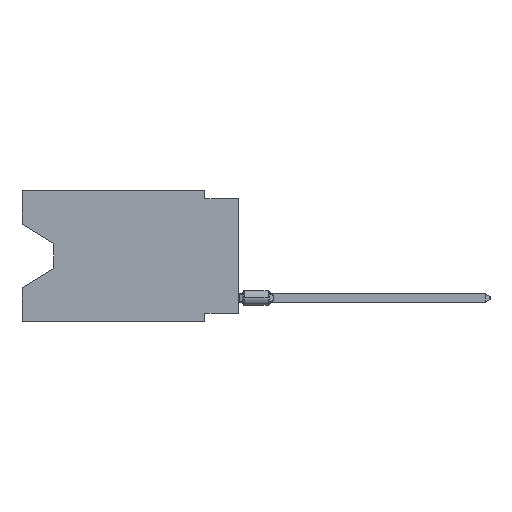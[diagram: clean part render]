
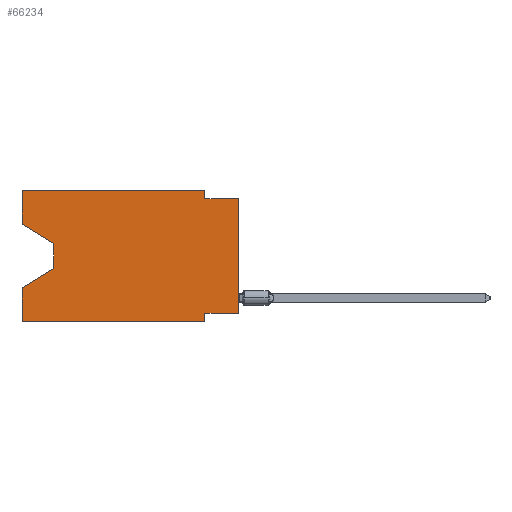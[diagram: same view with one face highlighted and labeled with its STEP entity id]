
A CAD part, left-side view. The second image highlights one B-rep face of the part: STEP entity #66234.
In plain terms, the highlighted planar face has unit normal (-1, 0, 0).
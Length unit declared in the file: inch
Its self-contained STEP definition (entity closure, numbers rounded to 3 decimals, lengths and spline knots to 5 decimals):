
#13 = DIRECTION ( 'NONE',  ( 0., -0.855, -0.519 ) ) ;
#1973 = DIRECTION ( 'NONE',  ( 0., -1., 0. ) ) ;
#2079 = EDGE_CURVE ( 'NONE', #6070, #27769, #16636, .T. ) ;
#2170 = EDGE_CURVE ( 'NONE', #6070, #48036, #61085, .T. ) ;
#4912 = DIRECTION ( 'NONE',  ( 0., 0., 1. ) ) ;
#6001 = CARTESIAN_POINT ( 'NONE',  ( 0., 0., 0. ) ) ;
#6070 = VERTEX_POINT ( 'NONE', #34363 ) ;
#8718 = CARTESIAN_POINT ( 'NONE',  ( 0., 0.645, 0. ) ) ;
#9773 = DIRECTION ( 'NONE',  ( 0., -1., 0. ) ) ;
#10427 = VECTOR ( 'NONE', #58293, 39.37008 ) ;
#11369 = CARTESIAN_POINT ( 'NONE',  ( 0., 0.645, -0.10025 ) ) ;
#11467 = DIRECTION ( 'NONE',  ( 0., 1., 0. ) ) ;
#11790 = VERTEX_POINT ( 'NONE', #64681 ) ;
#13899 = CARTESIAN_POINT ( 'NONE',  ( 0., 0., -0.025 ) ) ;
#14241 = LINE ( 'NONE', #26767, #72874 ) ;
#14348 = VERTEX_POINT ( 'NONE', #54433 ) ;
#14787 = VERTEX_POINT ( 'NONE', #48953 ) ;
#14793 = FACE_OUTER_BOUND ( 'NONE', #17022, .T. ) ;
#14929 = DIRECTION ( 'NONE',  ( 0., 0., -1. ) ) ;
#15572 = DIRECTION ( 'NONE',  ( 0., 0., -1. ) ) ;
#16636 = LINE ( 'NONE', #78474, #10427 ) ;
#16924 = DIRECTION ( 'NONE',  ( 0., 0., 1. ) ) ;
#17022 = EDGE_LOOP ( 'NONE', ( #77737, #52090, #46063, #29889, #41522, #38681, #74377, #63121, #40506, #45290, #59049, #35788 ) ) ;
#21013 = DIRECTION ( 'NONE',  ( 0., 0., -1. ) ) ;
#21389 = EDGE_CURVE ( 'NONE', #25518, #65332, #34711, .T. ) ;
#23384 = VECTOR ( 'NONE', #11467, 39.37008 ) ;
#24010 = CARTESIAN_POINT ( 'NONE',  ( 0., 0., -0.365 ) ) ;
#24041 = CARTESIAN_POINT ( 'NONE',  ( 0., 0., -0.365 ) ) ;
#25518 = VERTEX_POINT ( 'NONE', #32060 ) ;
#26013 = DIRECTION ( 'NONE',  ( 0., -1., 0. ) ) ;
#26548 = VERTEX_POINT ( 'NONE', #24041 ) ;
#26767 = CARTESIAN_POINT ( 'NONE',  ( 0., 0.645, -0.39 ) ) ;
#27011 = LINE ( 'NONE', #32675, #67946 ) ;
#27769 = VERTEX_POINT ( 'NONE', #66499 ) ;
#29889 = ORIENTED_EDGE ( 'NONE', *, *, #64045, .F. ) ;
#32060 = CARTESIAN_POINT ( 'NONE',  ( 0., 0.1, 0. ) ) ;
#32675 = CARTESIAN_POINT ( 'NONE',  ( 0., 0.645, 0. ) ) ;
#33351 = DIRECTION ( 'NONE',  ( 1., 0., 0. ) ) ;
#33460 = EDGE_CURVE ( 'NONE', #77255, #78059, #77399, .T. ) ;
#34363 = CARTESIAN_POINT ( 'NONE',  ( 0., 0.645, -0.10025 ) ) ;
#34711 = LINE ( 'NONE', #76390, #42936 ) ;
#35319 = CARTESIAN_POINT ( 'NONE',  ( 0., 0.645, -0.28975 ) ) ;
#35788 = ORIENTED_EDGE ( 'NONE', *, *, #2079, .F. ) ;
#37312 = CARTESIAN_POINT ( 'NONE',  ( 0., 0.1, -0.025 ) ) ;
#37750 = EDGE_CURVE ( 'NONE', #27769, #25518, #27011, .T. ) ;
#38680 = VECTOR ( 'NONE', #26013, 39.37008 ) ;
#38681 = ORIENTED_EDGE ( 'NONE', *, *, #68670, .F. ) ;
#39824 = VECTOR ( 'NONE', #4912, 39.37008 ) ;
#40506 = ORIENTED_EDGE ( 'NONE', *, *, #54333, .F. ) ;
#41522 = ORIENTED_EDGE ( 'NONE', *, *, #59738, .T. ) ;
#41677 = LINE ( 'NONE', #66348, #39824 ) ;
#42936 = VECTOR ( 'NONE', #21013, 39.37008 ) ;
#43378 = EDGE_CURVE ( 'NONE', #26548, #14348, #66836, .T. ) ;
#45290 = ORIENTED_EDGE ( 'NONE', *, *, #21389, .F. ) ;
#46063 = ORIENTED_EDGE ( 'NONE', *, *, #33460, .T. ) ;
#46192 = LINE ( 'NONE', #13899, #38680 ) ;
#46269 = DIRECTION ( 'NONE',  ( 0., 0., -1. ) ) ;
#47081 = CARTESIAN_POINT ( 'NONE',  ( 0., 0.55, -0.158 ) ) ;
#47676 = VECTOR ( 'NONE', #63695, 39.37008 ) ;
#48036 = VERTEX_POINT ( 'NONE', #68270 ) ;
#48953 = CARTESIAN_POINT ( 'NONE',  ( 0., 0.1, -0.39 ) ) ;
#51961 = CARTESIAN_POINT ( 'NONE',  ( 0., 0.55, -0.232 ) ) ;
#52090 = ORIENTED_EDGE ( 'NONE', *, *, #62322, .T. ) ;
#52495 = LINE ( 'NONE', #64608, #67225 ) ;
#52533 = CARTESIAN_POINT ( 'NONE',  ( 0., 0.645, -0.39 ) ) ;
#54333 = EDGE_CURVE ( 'NONE', #65332, #11790, #46192, .T. ) ;
#54433 = CARTESIAN_POINT ( 'NONE',  ( 0., 0.1, -0.365 ) ) ;
#54611 = CARTESIAN_POINT ( 'NONE',  ( 0., 0.55, -0.232 ) ) ;
#56183 = VECTOR ( 'NONE', #46269, 39.37008 ) ;
#58293 = DIRECTION ( 'NONE',  ( 0., 0., 1. ) ) ;
#59049 = ORIENTED_EDGE ( 'NONE', *, *, #37750, .F. ) ;
#59738 = EDGE_CURVE ( 'NONE', #61241, #14787, #14241, .T. ) ;
#61085 = LINE ( 'NONE', #11369, #76272 ) ;
#61241 = VERTEX_POINT ( 'NONE', #52533 ) ;
#61379 = LINE ( 'NONE', #6001, #64600 ) ;
#62063 = AXIS2_PLACEMENT_3D ( 'NONE', #8718, #33351, #15572 ) ;
#62322 = EDGE_CURVE ( 'NONE', #48036, #77255, #78584, .T. ) ;
#63121 = ORIENTED_EDGE ( 'NONE', *, *, #77773, .T. ) ;
#63695 = DIRECTION ( 'NONE',  ( 0., 0.855, -0.519 ) ) ;
#64045 = EDGE_CURVE ( 'NONE', #61241, #78059, #41677, .T. ) ;
#64600 = VECTOR ( 'NONE', #16924, 39.37008 ) ;
#64608 = CARTESIAN_POINT ( 'NONE',  ( 0., 0.1, -0.39 ) ) ;
#64681 = CARTESIAN_POINT ( 'NONE',  ( 0., 0., -0.025 ) ) ;
#65332 = VERTEX_POINT ( 'NONE', #37312 ) ;
#66234 = ADVANCED_FACE ( 'NONE', ( #14793 ), #77393, .F. ) ;
#66348 = CARTESIAN_POINT ( 'NONE',  ( 0., 0.645, 0. ) ) ;
#66499 = CARTESIAN_POINT ( 'NONE',  ( 0., 0.645, 0. ) ) ;
#66836 = LINE ( 'NONE', #24010, #23384 ) ;
#67225 = VECTOR ( 'NONE', #14929, 39.37008 ) ;
#67946 = VECTOR ( 'NONE', #1973, 39.37008 ) ;
#68270 = CARTESIAN_POINT ( 'NONE',  ( 0., 0.55, -0.158 ) ) ;
#68670 = EDGE_CURVE ( 'NONE', #14348, #14787, #52495, .T. ) ;
#72874 = VECTOR ( 'NONE', #9773, 39.37008 ) ;
#74377 = ORIENTED_EDGE ( 'NONE', *, *, #43378, .F. ) ;
#76272 = VECTOR ( 'NONE', #13, 39.37008 ) ;
#76390 = CARTESIAN_POINT ( 'NONE',  ( 0., 0.1, 0. ) ) ;
#77255 = VERTEX_POINT ( 'NONE', #54611 ) ;
#77393 = PLANE ( 'NONE',  #62063 ) ;
#77399 = LINE ( 'NONE', #51961, #47676 ) ;
#77737 = ORIENTED_EDGE ( 'NONE', *, *, #2170, .T. ) ;
#77773 = EDGE_CURVE ( 'NONE', #26548, #11790, #61379, .T. ) ;
#78059 = VERTEX_POINT ( 'NONE', #35319 ) ;
#78474 = CARTESIAN_POINT ( 'NONE',  ( 0., 0.645, 0. ) ) ;
#78584 = LINE ( 'NONE', #47081, #56183 ) ;
